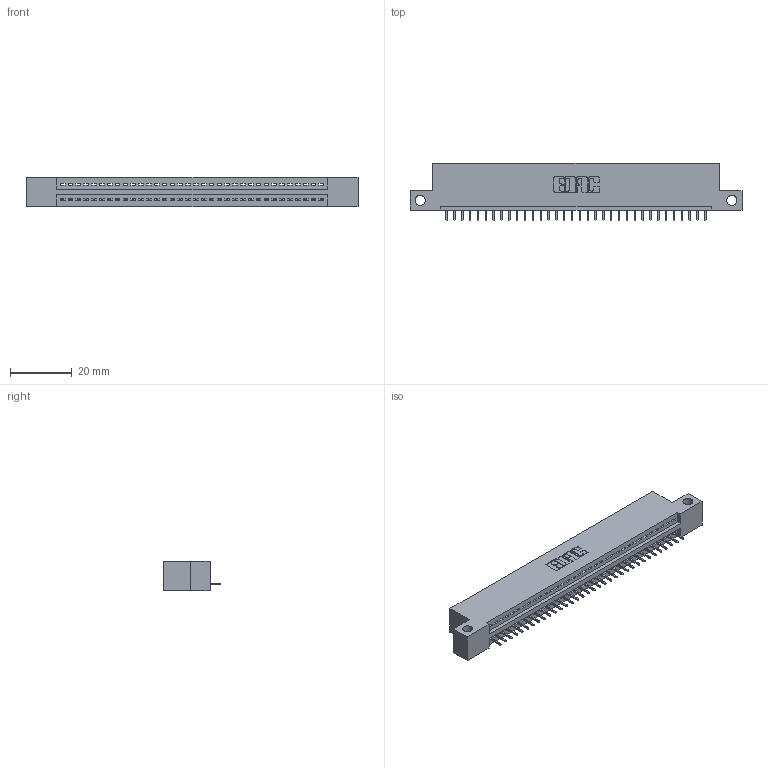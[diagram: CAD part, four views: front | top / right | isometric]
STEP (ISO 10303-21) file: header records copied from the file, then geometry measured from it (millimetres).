
FILE_DESCRIPTION (( 'STEP AP203' ), '1' );
FILE_NAME ('345-034-525-112.STEP', '2020-09-19T15:05:02', ( '' ), ( '' ), 'SwSTEP 2.0', 'SolidWorks 2020', '' );
FILE_SCHEMA (( 'CONFIG_CONTROL_DESIGN' ));
Length unit declared in the file: inch
Products named in the file (3): 345 Part_Flush Mounting Lugs - Side Mount; 345-034-525-112; 345-292-001_345-293-125
Assembly tree (35 placements, depth 2):
  345-034-525-112
    345 Part_Flush Mounting Lugs - Side Mount
    345-292-001_345-293-125  x34
Bounding box: 107.57 x 18.72 x 9.4 mm (x, y, z)
Volume: 9925.4 mm3; surface area: 12476.3 mm2
Topology: 35 solids, 35 shells, 2234 faces, 6461 edges, 4170 vertices
Faces by surface type: plane 1644, cylinder 590
Entity records: 26743 total; most frequent: CARTESIAN_POINT 4638, ORIENTED_EDGE 4606, DIRECTION 4063, EDGE_CURVE 2303, LINE 2039, VECTOR 2039, VERTEX_POINT 1530, AXIS2_PLACEMENT_3D 1012
